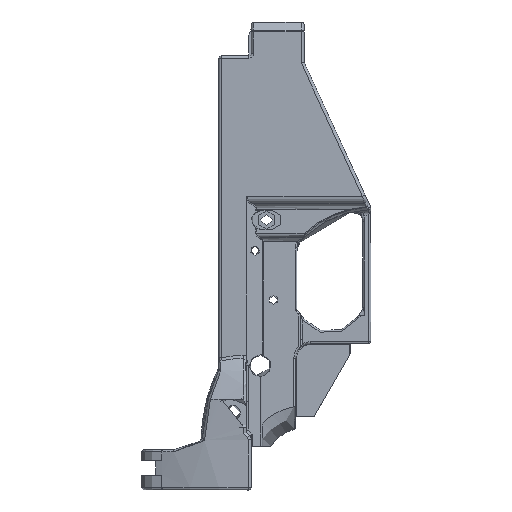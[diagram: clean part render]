
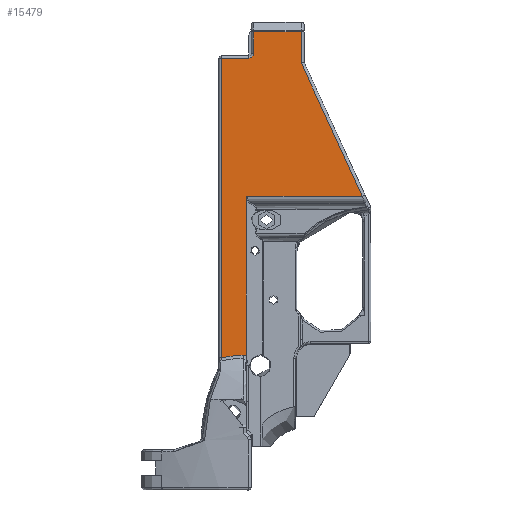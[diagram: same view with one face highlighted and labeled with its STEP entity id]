
A CAD part, left-side view. The second image highlights one B-rep face of the part: STEP entity #15479.
In plain terms, the highlighted planar face has unit normal (-1, 0, 0).
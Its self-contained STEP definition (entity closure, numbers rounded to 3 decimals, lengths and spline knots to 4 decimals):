
#221=ELLIPSE('',#16887,1.9201,1.636);
#397=PLANE('',#16885);
#1357=FACE_OUTER_BOUND('',#2308,.T.);
#2308=EDGE_LOOP('',(#12529,#12530,#12531,#12532,#12533,#12534,#12535,#12536,
#12537,#12538,#12539,#12540));
#3251=B_SPLINE_CURVE_WITH_KNOTS('',3,(#43739,#43740,#43741,#43742),
 .UNSPECIFIED.,.F.,.F.,(4,4),(-0.1434,0.),
 .UNSPECIFIED.);
#3252=B_SPLINE_CURVE_WITH_KNOTS('',3,(#43746,#43747,#43748,#43749,#43750,
#43751,#43752,#43753,#43754,#43755,#43756,#43757),.UNSPECIFIED.,.F.,.F.,
(4,2,2,2,2,4),(-0.117,-0.1147,-0.0798,
-0.057,-0.0072,0.),.UNSPECIFIED.);
#3886=CIRCLE('',#16886,0.08);
#4506=LINE('',#26275,#5275);
#4508=LINE('',#26306,#5277);
#4688=LINE('',#43691,#5457);
#4692=LINE('',#43729,#5461);
#4693=LINE('',#43733,#5462);
#4694=LINE('',#43735,#5463);
#4695=LINE('',#43744,#5464);
#4696=LINE('',#43758,#5465);
#5275=VECTOR('',#19141,0.3937);
#5277=VECTOR('',#19153,0.3937);
#5457=VECTOR('',#19977,0.3937);
#5461=VECTOR('',#19999,0.3937);
#5462=VECTOR('',#20002,0.3937);
#5463=VECTOR('',#20003,0.3937);
#5464=VECTOR('',#20006,1.6985);
#5465=VECTOR('',#20007,0.1181);
#6299=VERTEX_POINT('',#26272);
#6300=VERTEX_POINT('',#26274);
#6304=VERTEX_POINT('',#26304);
#6804=VERTEX_POINT('',#43689);
#6809=VERTEX_POINT('',#43728);
#6810=VERTEX_POINT('',#43730);
#6811=VERTEX_POINT('',#43732);
#6812=VERTEX_POINT('',#43734);
#6813=VERTEX_POINT('',#43736);
#6814=VERTEX_POINT('',#43738);
#6815=VERTEX_POINT('',#43743);
#6816=VERTEX_POINT('',#43745);
#8097=EDGE_CURVE('',#6299,#6300,#4506,.T.);
#8104=EDGE_CURVE('',#6304,#6299,#4508,.T.);
#8837=EDGE_CURVE('',#6804,#6304,#4688,.T.);
#8846=EDGE_CURVE('',#6809,#6804,#4692,.T.);
#8847=EDGE_CURVE('',#6810,#6809,#3886,.T.);
#8848=EDGE_CURVE('',#6811,#6810,#4693,.T.);
#8849=EDGE_CURVE('',#6812,#6811,#4694,.T.);
#8850=EDGE_CURVE('',#6813,#6812,#221,.T.);
#8851=EDGE_CURVE('',#6814,#6813,#3251,.T.);
#8852=EDGE_CURVE('',#6815,#6814,#4695,.T.);
#8853=EDGE_CURVE('',#6816,#6815,#3252,.T.);
#8854=EDGE_CURVE('',#6300,#6816,#4696,.T.);
#12529=ORIENTED_EDGE('',*,*,#8097,.F.);
#12530=ORIENTED_EDGE('',*,*,#8104,.F.);
#12531=ORIENTED_EDGE('',*,*,#8837,.F.);
#12532=ORIENTED_EDGE('',*,*,#8846,.F.);
#12533=ORIENTED_EDGE('',*,*,#8847,.F.);
#12534=ORIENTED_EDGE('',*,*,#8848,.F.);
#12535=ORIENTED_EDGE('',*,*,#8849,.F.);
#12536=ORIENTED_EDGE('',*,*,#8850,.F.);
#12537=ORIENTED_EDGE('',*,*,#8851,.F.);
#12538=ORIENTED_EDGE('',*,*,#8852,.F.);
#12539=ORIENTED_EDGE('',*,*,#8853,.F.);
#12540=ORIENTED_EDGE('',*,*,#8854,.F.);
#15479=ADVANCED_FACE('',(#1357),#397,.F.);
#16885=AXIS2_PLACEMENT_3D('',#43727,#19997,#19998);
#16886=AXIS2_PLACEMENT_3D('',#43731,#20000,#20001);
#16887=AXIS2_PLACEMENT_3D('',#43737,#20004,#20005);
#19141=DIRECTION('',(0.,-0.417,-0.909));
#19153=DIRECTION('',(0.,0.,-1.));
#19977=DIRECTION('',(0.,-1.,0.));
#19997=DIRECTION('center_axis',(1.,0.,0.));
#19998=DIRECTION('ref_axis',(0.,0.,
-1.));
#19999=DIRECTION('',(0.,0.,1.));
#20000=DIRECTION('center_axis',(-1.,0.,0.));
#20001=DIRECTION('ref_axis',(0.,-0.707,-0.707));
#20002=DIRECTION('',(0.,-1.,0.));
#20003=DIRECTION('',(0.,0.,1.));
#20004=DIRECTION('center_axis',(-1.,0.,0.));
#20005=DIRECTION('ref_axis',(0.,-0.984,-0.179));
#20006=DIRECTION('',(0.,0.,-1.));
#20007=DIRECTION('',(0.,1.,0.));
#26272=CARTESIAN_POINT('',(-0.731,-0.0727,2.8507));
#26274=CARTESIAN_POINT('',(-0.731,-1.118,0.5717));
#26275=CARTESIAN_POINT('',(-0.731,-1.4648,-0.1846));
#26304=CARTESIAN_POINT('',(-0.731,-0.0728,3.3816));
#26306=CARTESIAN_POINT('',(-0.731,-0.0727,-0.2092));
#43689=CARTESIAN_POINT('',(-0.731,0.7372,3.3816));
#43691=CARTESIAN_POINT('',(-0.731,0.7121,3.3816));
#43727=CARTESIAN_POINT('Origin',(-0.731,0.68,-3.6849));
#43728=CARTESIAN_POINT('',(-0.731,0.7373,3.0095));
#43729=CARTESIAN_POINT('',(-0.731,0.7373,-0.0118));
#43730=CARTESIAN_POINT('',(-0.731,0.8173,2.9295));
#43731=CARTESIAN_POINT('Origin',(-0.731,0.8173,3.0095));
#43732=CARTESIAN_POINT('',(-0.731,1.2902,2.9295));
#43733=CARTESIAN_POINT('',(-0.731,0.7441,2.9295));
#43734=CARTESIAN_POINT('',(-0.731,1.2902,-2.1813));
#43735=CARTESIAN_POINT('',(-0.731,1.2902,-3.1756));
#43736=CARTESIAN_POINT('',(-0.731,0.9158,-2.1342));
#43737=CARTESIAN_POINT('Origin',(-0.731,0.7244,-3.7785));
#43738=CARTESIAN_POINT('',(-0.731,0.8628,-2.151));
#43739=CARTESIAN_POINT('Ctrl Pts',(-0.731,0.8629,
-2.151));
#43740=CARTESIAN_POINT('Ctrl Pts',(-0.731,0.8784,
-2.1404));
#43741=CARTESIAN_POINT('Ctrl Pts',(-0.731,0.8969,
-2.1335));
#43742=CARTESIAN_POINT('Ctrl Pts',(-0.731,0.9158,
-2.1342));
#43743=CARTESIAN_POINT('',(-0.731,0.8628,0.5319));
#43744=CARTESIAN_POINT('',(-0.731,0.8628,-2.5001));
#43745=CARTESIAN_POINT('',(-0.731,0.8546,0.5717));
#43746=CARTESIAN_POINT('Ctrl Pts',(-0.731,0.8546,
0.5717));
#43747=CARTESIAN_POINT('Ctrl Pts',(-0.731,0.8546,
0.5716));
#43748=CARTESIAN_POINT('Ctrl Pts',(-0.731,0.8546,
0.5716));
#43749=CARTESIAN_POINT('Ctrl Pts',(-0.731,0.855,
0.5706));
#43750=CARTESIAN_POINT('Ctrl Pts',(-0.731,0.8564,
0.5674));
#43751=CARTESIAN_POINT('Ctrl Pts',(-0.731,0.8587,
0.5601));
#43752=CARTESIAN_POINT('Ctrl Pts',(-0.731,0.8595,
0.5572));
#43753=CARTESIAN_POINT('Ctrl Pts',(-0.731,0.8617,
0.5478));
#43754=CARTESIAN_POINT('Ctrl Pts',(-0.731,0.8626,
0.5413));
#43755=CARTESIAN_POINT('Ctrl Pts',(-0.731,0.8628,
0.5338));
#43756=CARTESIAN_POINT('Ctrl Pts',(-0.731,0.8628,
0.5329));
#43757=CARTESIAN_POINT('Ctrl Pts',(-0.731,0.8628,
0.5319));
#43758=CARTESIAN_POINT('',(-0.731,1.0895,0.5717));
